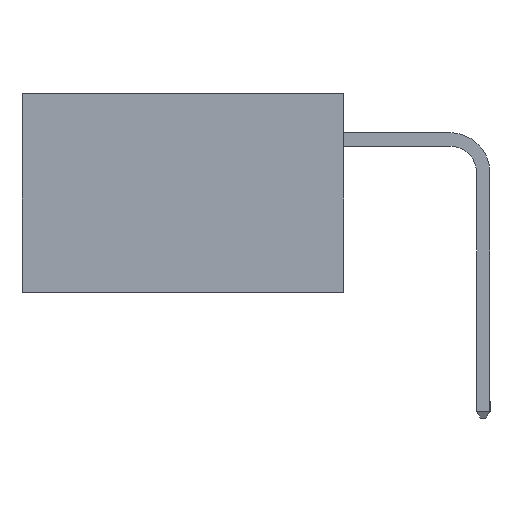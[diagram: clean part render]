
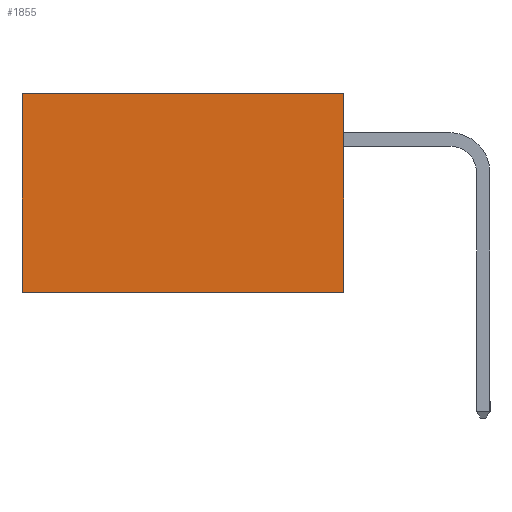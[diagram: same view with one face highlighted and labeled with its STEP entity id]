
A CAD part, left-side view. The second image highlights one B-rep face of the part: STEP entity #1855.
In plain terms, the highlighted planar face has unit normal (-1, 0, 0).
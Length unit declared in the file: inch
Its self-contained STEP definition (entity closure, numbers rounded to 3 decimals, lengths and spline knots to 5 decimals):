
#2 = LINE ( 'NONE', #11384, #9727 ) ;
#7 = DIRECTION ( 'NONE',  ( 0., 1., 0. ) ) ;
#17 = EDGE_CURVE ( 'NONE', #7862, #4307, #2, .T. ) ;
#274 = AXIS2_PLACEMENT_3D ( 'NONE', #9522, #10552, #5439 ) ;
#1671 = LINE ( 'NONE', #7321, #5862 ) ;
#1855 = ADVANCED_FACE ( 'NONE', ( #8238 ), #2268, .F. ) ;
#2268 = PLANE ( 'NONE',  #274 ) ;
#2293 = ORIENTED_EDGE ( 'NONE', *, *, #7318, .F. ) ;
#3485 = CARTESIAN_POINT ( 'NONE',  ( 0.2615, 0.6, 0. ) ) ;
#3938 = VERTEX_POINT ( 'NONE', #9747 ) ;
#4167 = CARTESIAN_POINT ( 'NONE',  ( 0.2615, 0., 0. ) ) ;
#4307 = VERTEX_POINT ( 'NONE', #6761 ) ;
#4850 = DIRECTION ( 'NONE',  ( 0., 0., -1. ) ) ;
#4992 = ORIENTED_EDGE ( 'NONE', *, *, #17, .T. ) ;
#5183 = DIRECTION ( 'NONE',  ( 0., 1., 0. ) ) ;
#5212 = VECTOR ( 'NONE', #4850, 39.37008 ) ;
#5439 = DIRECTION ( 'NONE',  ( 0., 0., -1. ) ) ;
#5862 = VECTOR ( 'NONE', #5183, 39.37008 ) ;
#6116 = EDGE_CURVE ( 'NONE', #3938, #7862, #8988, .T. ) ;
#6361 = VERTEX_POINT ( 'NONE', #12941 ) ;
#6761 = CARTESIAN_POINT ( 'NONE',  ( 0.2615, 0.6, -0.37 ) ) ;
#7318 = EDGE_CURVE ( 'NONE', #6361, #4307, #1671, .T. ) ;
#7321 = CARTESIAN_POINT ( 'NONE',  ( 0.2615, 0., -0.37 ) ) ;
#7862 = VERTEX_POINT ( 'NONE', #3485 ) ;
#8113 = EDGE_LOOP ( 'NONE', ( #4992, #2293, #12724, #9110 ) ) ;
#8238 = FACE_OUTER_BOUND ( 'NONE', #8113, .T. ) ;
#8988 = LINE ( 'NONE', #4167, #11616 ) ;
#9110 = ORIENTED_EDGE ( 'NONE', *, *, #6116, .T. ) ;
#9522 = CARTESIAN_POINT ( 'NONE',  ( 0.2615, 0., -0.37 ) ) ;
#9727 = VECTOR ( 'NONE', #11438, 39.37008 ) ;
#9747 = CARTESIAN_POINT ( 'NONE',  ( 0.2615, 0., 0. ) ) ;
#10552 = DIRECTION ( 'NONE',  ( 1., 0., 0. ) ) ;
#11380 = LINE ( 'NONE', #11797, #5212 ) ;
#11384 = CARTESIAN_POINT ( 'NONE',  ( 0.2615, 0.6, -0.37 ) ) ;
#11438 = DIRECTION ( 'NONE',  ( 0., 0., -1. ) ) ;
#11616 = VECTOR ( 'NONE', #7, 39.37008 ) ;
#11797 = CARTESIAN_POINT ( 'NONE',  ( 0.2615, 0., -0.37 ) ) ;
#11971 = EDGE_CURVE ( 'NONE', #3938, #6361, #11380, .T. ) ;
#12724 = ORIENTED_EDGE ( 'NONE', *, *, #11971, .F. ) ;
#12941 = CARTESIAN_POINT ( 'NONE',  ( 0.2615, 0., -0.37 ) ) ;
